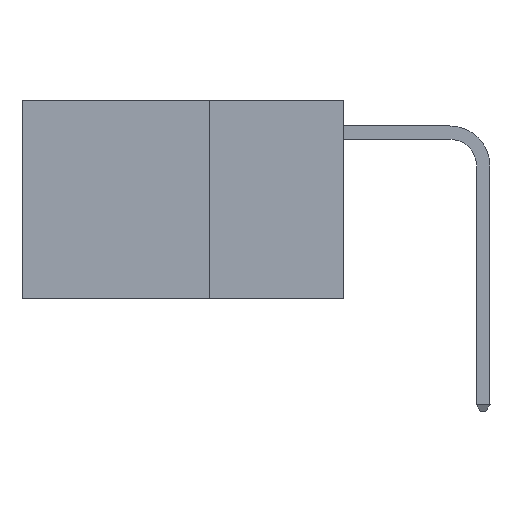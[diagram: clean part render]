
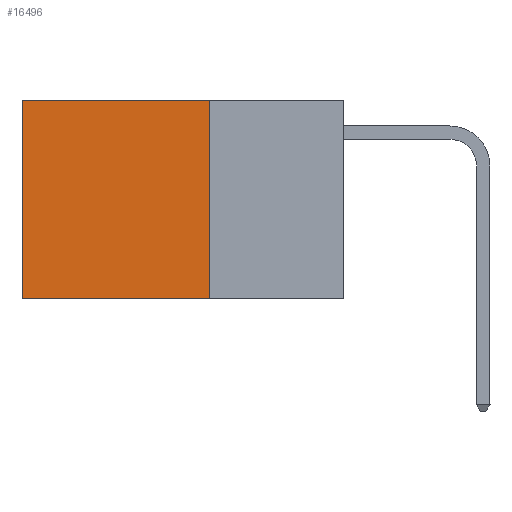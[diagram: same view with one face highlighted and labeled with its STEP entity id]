
A CAD part, left-side view. The second image highlights one B-rep face of the part: STEP entity #16496.
In plain terms, the highlighted planar face has unit normal (-1, 0, 0).
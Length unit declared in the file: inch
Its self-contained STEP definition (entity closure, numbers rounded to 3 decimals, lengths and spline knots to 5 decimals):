
#37 = VECTOR ( 'NONE', #12023, 39.37008 ) ;
#410 = ORIENTED_EDGE ( 'NONE', *, *, #17999, .F. ) ;
#825 = VECTOR ( 'NONE', #10513, 39.37008 ) ;
#926 = EDGE_LOOP ( 'NONE', ( #8774, #11681, #410, #21814 ) ) ;
#1322 = VERTEX_POINT ( 'NONE', #16116 ) ;
#1659 = VERTEX_POINT ( 'NONE', #13460 ) ;
#2246 = PLANE ( 'NONE',  #22945 ) ;
#4096 = EDGE_CURVE ( 'NONE', #1322, #12637, #16380, .T. ) ;
#6049 = CARTESIAN_POINT ( 'NONE',  ( 0.2625, 0.25, 0. ) ) ;
#7026 = FACE_OUTER_BOUND ( 'NONE', #926, .T. ) ;
#7243 = CARTESIAN_POINT ( 'NONE',  ( 0.2625, 0.6, 0. ) ) ;
#7946 = DIRECTION ( 'NONE',  ( 0., 0., -1. ) ) ;
#8774 = ORIENTED_EDGE ( 'NONE', *, *, #8882, .T. ) ;
#8882 = EDGE_CURVE ( 'NONE', #13071, #12637, #12365, .T. ) ;
#8963 = VECTOR ( 'NONE', #12149, 39.37008 ) ;
#9123 = DIRECTION ( 'NONE',  ( 0., 0., -1. ) ) ;
#10513 = DIRECTION ( 'NONE',  ( 0., 1., 0. ) ) ;
#11681 = ORIENTED_EDGE ( 'NONE', *, *, #4096, .F. ) ;
#12023 = DIRECTION ( 'NONE',  ( 0., 1., 0. ) ) ;
#12149 = DIRECTION ( 'NONE',  ( 0., 0., -1. ) ) ;
#12365 = LINE ( 'NONE', #7243, #17300 ) ;
#12637 = VERTEX_POINT ( 'NONE', #13411 ) ;
#13071 = VERTEX_POINT ( 'NONE', #20431 ) ;
#13411 = CARTESIAN_POINT ( 'NONE',  ( 0.2625, 0.6, -0.37 ) ) ;
#13460 = CARTESIAN_POINT ( 'NONE',  ( 0.2625, 0.25, 0. ) ) ;
#14603 = EDGE_CURVE ( 'NONE', #1659, #13071, #20581, .T. ) ;
#16116 = CARTESIAN_POINT ( 'NONE',  ( 0.2625, 0.25, -0.37 ) ) ;
#16380 = LINE ( 'NONE', #17932, #825 ) ;
#16496 = ADVANCED_FACE ( 'NONE', ( #7026 ), #2246, .F. ) ;
#17300 = VECTOR ( 'NONE', #9123, 39.37008 ) ;
#17932 = CARTESIAN_POINT ( 'NONE',  ( 0.2625, 0.25, -0.37 ) ) ;
#17999 = EDGE_CURVE ( 'NONE', #1659, #1322, #20085, .T. ) ;
#19129 = DIRECTION ( 'NONE',  ( 1., 0., 0. ) ) ;
#20085 = LINE ( 'NONE', #21440, #8963 ) ;
#20431 = CARTESIAN_POINT ( 'NONE',  ( 0.2625, 0.6, 0. ) ) ;
#20581 = LINE ( 'NONE', #21322, #37 ) ;
#21322 = CARTESIAN_POINT ( 'NONE',  ( 0.2625, 0.25, 0. ) ) ;
#21440 = CARTESIAN_POINT ( 'NONE',  ( 0.2625, 0.25, 0. ) ) ;
#21814 = ORIENTED_EDGE ( 'NONE', *, *, #14603, .T. ) ;
#22945 = AXIS2_PLACEMENT_3D ( 'NONE', #6049, #19129, #7946 ) ;
